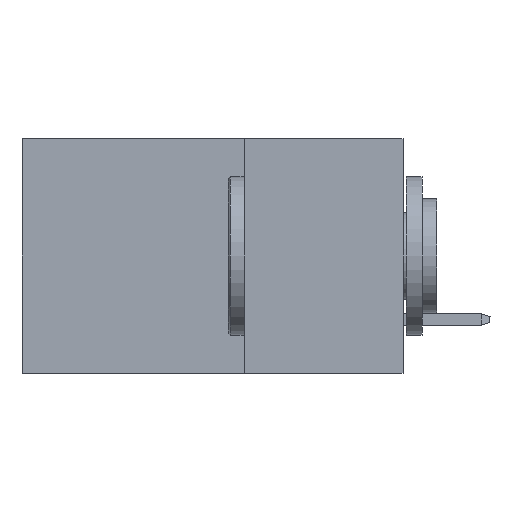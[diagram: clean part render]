
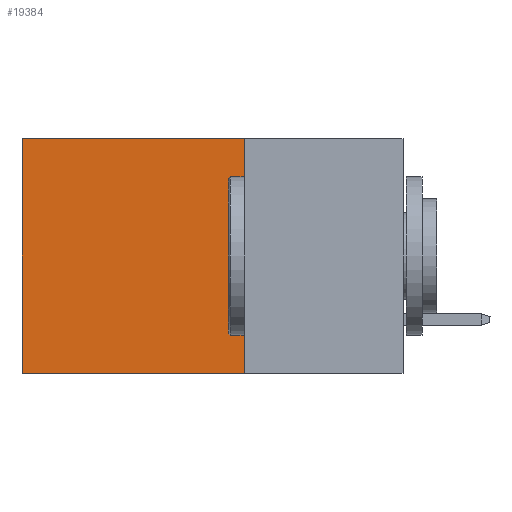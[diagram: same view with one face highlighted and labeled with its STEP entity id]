
A CAD part, left-side view. The second image highlights one B-rep face of the part: STEP entity #19384.
In plain terms, the highlighted planar face has unit normal (-1, 0, 0).
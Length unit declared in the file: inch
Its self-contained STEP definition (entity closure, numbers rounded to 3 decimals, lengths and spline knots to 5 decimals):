
#181 = VECTOR ( 'NONE', #7126, 39.37008 ) ;
#1784 = EDGE_CURVE ( 'NONE', #18851, #17236, #25185, .T. ) ;
#2271 = LINE ( 'NONE', #4495, #27981 ) ;
#2946 = CARTESIAN_POINT ( 'NONE',  ( 0.2875, 0.25, 0. ) ) ;
#3092 = VERTEX_POINT ( 'NONE', #5173 ) ;
#4495 = CARTESIAN_POINT ( 'NONE',  ( 0.2875, 0.25, 0. ) ) ;
#4642 = VECTOR ( 'NONE', #6409, 39.37008 ) ;
#5173 = CARTESIAN_POINT ( 'NONE',  ( 0.2875, 0.6, -0.37 ) ) ;
#5917 = LINE ( 'NONE', #8158, #28014 ) ;
#6409 = DIRECTION ( 'NONE',  ( 0., 1., 0. ) ) ;
#7126 = DIRECTION ( 'NONE',  ( 0., 1., 0. ) ) ;
#8158 = CARTESIAN_POINT ( 'NONE',  ( 0.2875, 0.6, 0. ) ) ;
#8636 = AXIS2_PLACEMENT_3D ( 'NONE', #21215, #23153, #23735 ) ;
#8815 = ORIENTED_EDGE ( 'NONE', *, *, #29076, .T. ) ;
#9006 = ORIENTED_EDGE ( 'NONE', *, *, #1784, .T. ) ;
#11231 = CARTESIAN_POINT ( 'NONE',  ( 0.2875, 0.25, 0. ) ) ;
#11317 = ORIENTED_EDGE ( 'NONE', *, *, #19189, .F. ) ;
#13292 = CARTESIAN_POINT ( 'NONE',  ( 0.2875, 0.25, -0.37 ) ) ;
#13991 = EDGE_CURVE ( 'NONE', #18678, #3092, #26695, .T. ) ;
#15269 = DIRECTION ( 'NONE',  ( 0., 0., -1. ) ) ;
#17236 = VERTEX_POINT ( 'NONE', #19389 ) ;
#18297 = EDGE_LOOP ( 'NONE', ( #8815, #25920, #11317, #9006 ) ) ;
#18678 = VERTEX_POINT ( 'NONE', #13292 ) ;
#18851 = VERTEX_POINT ( 'NONE', #11231 ) ;
#19189 = EDGE_CURVE ( 'NONE', #18851, #18678, #2271, .T. ) ;
#19384 = ADVANCED_FACE ( 'NONE', ( #23304 ), #27900, .F. ) ;
#19389 = CARTESIAN_POINT ( 'NONE',  ( 0.2875, 0.6, 0. ) ) ;
#21215 = CARTESIAN_POINT ( 'NONE',  ( 0.2875, 0.25, 0. ) ) ;
#23153 = DIRECTION ( 'NONE',  ( 1., 0., 0. ) ) ;
#23304 = FACE_OUTER_BOUND ( 'NONE', #18297, .T. ) ;
#23735 = DIRECTION ( 'NONE',  ( 0., 0., -1. ) ) ;
#25185 = LINE ( 'NONE', #2946, #181 ) ;
#25240 = DIRECTION ( 'NONE',  ( 0., 0., -1. ) ) ;
#25920 = ORIENTED_EDGE ( 'NONE', *, *, #13991, .F. ) ;
#26695 = LINE ( 'NONE', #26976, #4642 ) ;
#26976 = CARTESIAN_POINT ( 'NONE',  ( 0.2875, 0.25, -0.37 ) ) ;
#27900 = PLANE ( 'NONE',  #8636 ) ;
#27981 = VECTOR ( 'NONE', #25240, 39.37008 ) ;
#28014 = VECTOR ( 'NONE', #15269, 39.37008 ) ;
#29076 = EDGE_CURVE ( 'NONE', #17236, #3092, #5917, .T. ) ;
